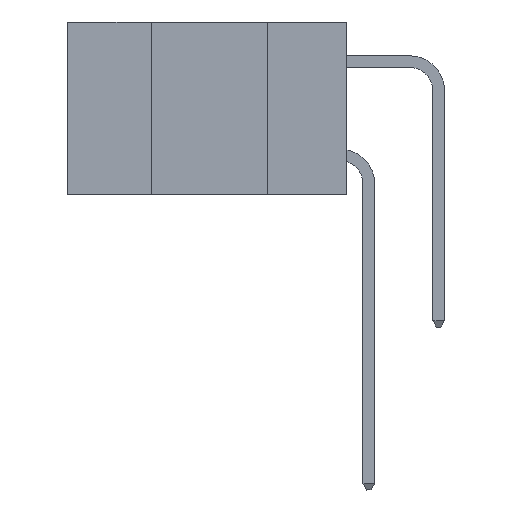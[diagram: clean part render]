
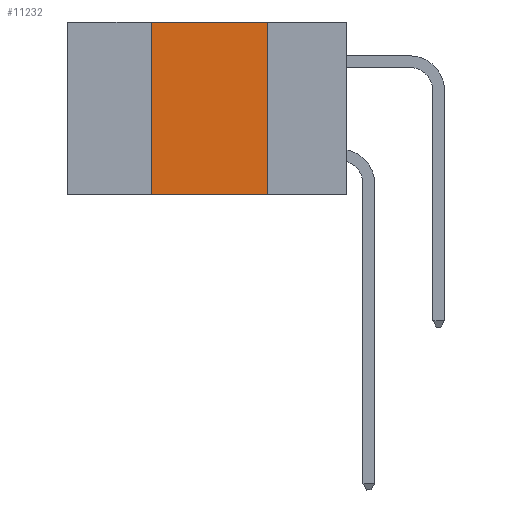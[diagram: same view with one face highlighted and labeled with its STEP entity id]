
A CAD part, left-side view. The second image highlights one B-rep face of the part: STEP entity #11232.
In plain terms, the highlighted planar face has unit normal (-1, 0, 0).
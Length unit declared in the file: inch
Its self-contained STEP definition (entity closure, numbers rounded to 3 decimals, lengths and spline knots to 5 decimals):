
#477 = EDGE_CURVE ( 'NONE', #10704, #18817, #20897, .T. ) ;
#864 = VECTOR ( 'NONE', #13388, 39.37008 ) ;
#2241 = VECTOR ( 'NONE', #2612, 39.37008 ) ;
#2487 = DIRECTION ( 'NONE',  ( 0., 0., -1. ) ) ;
#2497 = EDGE_CURVE ( 'NONE', #18817, #20857, #15715, .T. ) ;
#2612 = DIRECTION ( 'NONE',  ( 0., 0., -1. ) ) ;
#4055 = DIRECTION ( 'NONE',  ( 0., -1., 0. ) ) ;
#4619 = DIRECTION ( 'NONE',  ( 1., 0., 0. ) ) ;
#5518 = ORIENTED_EDGE ( 'NONE', *, *, #477, .F. ) ;
#6389 = PLANE ( 'NONE',  #25728 ) ;
#6486 = CARTESIAN_POINT ( 'NONE',  ( 0., 0.6, 0. ) ) ;
#6698 = EDGE_CURVE ( 'NONE', #20857, #18644, #13645, .T. ) ;
#10592 = EDGE_LOOP ( 'NONE', ( #20581, #18195, #5518, #25706 ) ) ;
#10704 = VERTEX_POINT ( 'NONE', #14836 ) ;
#11053 = FACE_OUTER_BOUND ( 'NONE', #10592, .T. ) ;
#11232 = ADVANCED_FACE ( 'NONE', ( #11053 ), #6389, .F. ) ;
#11279 = VECTOR ( 'NONE', #23201, 39.37008 ) ;
#12017 = CARTESIAN_POINT ( 'NONE',  ( 0., 0.6, -0.37 ) ) ;
#12811 = LINE ( 'NONE', #12017, #24910 ) ;
#13388 = DIRECTION ( 'NONE',  ( 0., 0., 1. ) ) ;
#13645 = LINE ( 'NONE', #18759, #2241 ) ;
#14231 = CARTESIAN_POINT ( 'NONE',  ( 0., 0.42, 0. ) ) ;
#14659 = CARTESIAN_POINT ( 'NONE',  ( 0., 0.17, 0. ) ) ;
#14836 = CARTESIAN_POINT ( 'NONE',  ( 0., 0.42, -0.37 ) ) ;
#15715 = LINE ( 'NONE', #25335, #11279 ) ;
#16882 = CARTESIAN_POINT ( 'NONE',  ( 0., 0.42, 0. ) ) ;
#18195 = ORIENTED_EDGE ( 'NONE', *, *, #2497, .F. ) ;
#18644 = VERTEX_POINT ( 'NONE', #19695 ) ;
#18759 = CARTESIAN_POINT ( 'NONE',  ( 0., 0.17, 0. ) ) ;
#18817 = VERTEX_POINT ( 'NONE', #14231 ) ;
#19695 = CARTESIAN_POINT ( 'NONE',  ( 0., 0.17, -0.37 ) ) ;
#20581 = ORIENTED_EDGE ( 'NONE', *, *, #6698, .F. ) ;
#20857 = VERTEX_POINT ( 'NONE', #14659 ) ;
#20897 = LINE ( 'NONE', #16882, #864 ) ;
#23201 = DIRECTION ( 'NONE',  ( 0., -1., 0. ) ) ;
#24910 = VECTOR ( 'NONE', #4055, 39.37008 ) ;
#25335 = CARTESIAN_POINT ( 'NONE',  ( 0., 0.6, 0. ) ) ;
#25706 = ORIENTED_EDGE ( 'NONE', *, *, #26024, .T. ) ;
#25728 = AXIS2_PLACEMENT_3D ( 'NONE', #6486, #4619, #2487 ) ;
#26024 = EDGE_CURVE ( 'NONE', #10704, #18644, #12811, .T. ) ;
